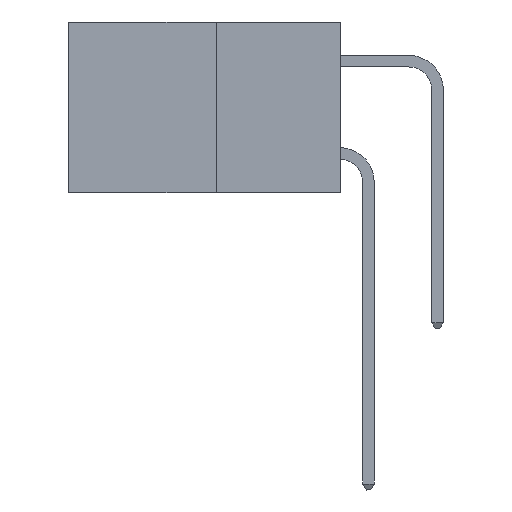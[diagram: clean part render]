
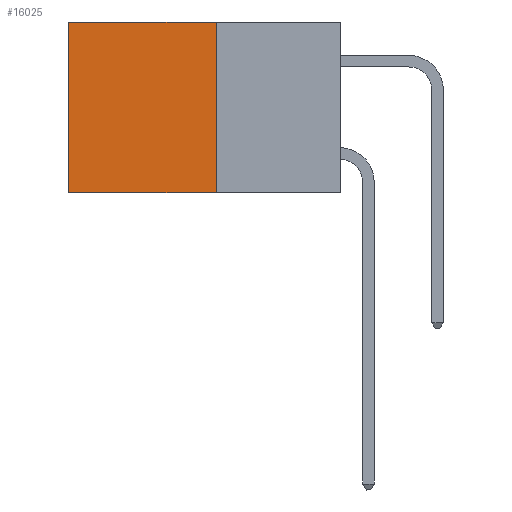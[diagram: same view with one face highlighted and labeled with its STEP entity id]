
A CAD part, left-side view. The second image highlights one B-rep face of the part: STEP entity #16025.
In plain terms, the highlighted planar face has unit normal (-1, 0, 0).
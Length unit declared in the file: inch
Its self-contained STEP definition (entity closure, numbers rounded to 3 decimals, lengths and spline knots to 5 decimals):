
#221 = EDGE_LOOP ( 'NONE', ( #6237, #7981, #3574, #17162 ) ) ;
#308 = CARTESIAN_POINT ( 'NONE',  ( 0.277, 0.59, -0.37 ) ) ;
#577 = EDGE_CURVE ( 'NONE', #3611, #1436, #14157, .T. ) ;
#1436 = VERTEX_POINT ( 'NONE', #17372 ) ;
#3574 = ORIENTED_EDGE ( 'NONE', *, *, #18549, .F. ) ;
#3611 = VERTEX_POINT ( 'NONE', #19410 ) ;
#4179 = DIRECTION ( 'NONE',  ( 0., 0., -1. ) ) ;
#4220 = DIRECTION ( 'NONE',  ( 1., 0., 0. ) ) ;
#4270 = PLANE ( 'NONE',  #16732 ) ;
#4299 = CARTESIAN_POINT ( 'NONE',  ( 0.277, 0.27, -0.37 ) ) ;
#4563 = EDGE_CURVE ( 'NONE', #4856, #1436, #8971, .T. ) ;
#4856 = VERTEX_POINT ( 'NONE', #14349 ) ;
#5514 = VECTOR ( 'NONE', #19115, 39.37008 ) ;
#5654 = VERTEX_POINT ( 'NONE', #15924 ) ;
#6237 = ORIENTED_EDGE ( 'NONE', *, *, #577, .T. ) ;
#6340 = FACE_OUTER_BOUND ( 'NONE', #221, .T. ) ;
#7776 = CARTESIAN_POINT ( 'NONE',  ( 0.277, 0.27, -0.37 ) ) ;
#7947 = CARTESIAN_POINT ( 'NONE',  ( 0.277, 0.27, -0.37 ) ) ;
#7981 = ORIENTED_EDGE ( 'NONE', *, *, #4563, .F. ) ;
#8590 = EDGE_CURVE ( 'NONE', #5654, #3611, #17774, .T. ) ;
#8971 = LINE ( 'NONE', #7776, #9439 ) ;
#8977 = DIRECTION ( 'NONE',  ( 0., 1., 0. ) ) ;
#9439 = VECTOR ( 'NONE', #16878, 39.37008 ) ;
#9458 = DIRECTION ( 'NONE',  ( 0., 0., -1. ) ) ;
#11848 = LINE ( 'NONE', #7947, #19123 ) ;
#13586 = VECTOR ( 'NONE', #8977, 39.37008 ) ;
#14157 = LINE ( 'NONE', #308, #5514 ) ;
#14349 = CARTESIAN_POINT ( 'NONE',  ( 0.277, 0.27, -0.37 ) ) ;
#15013 = CARTESIAN_POINT ( 'NONE',  ( 0.277, 0.27, 0. ) ) ;
#15924 = CARTESIAN_POINT ( 'NONE',  ( 0.277, 0.27, 0. ) ) ;
#16025 = ADVANCED_FACE ( 'NONE', ( #6340 ), #4270, .F. ) ;
#16732 = AXIS2_PLACEMENT_3D ( 'NONE', #4299, #4220, #4179 ) ;
#16878 = DIRECTION ( 'NONE',  ( 0., 1., 0. ) ) ;
#17162 = ORIENTED_EDGE ( 'NONE', *, *, #8590, .T. ) ;
#17372 = CARTESIAN_POINT ( 'NONE',  ( 0.277, 0.59, -0.37 ) ) ;
#17774 = LINE ( 'NONE', #15013, #13586 ) ;
#18549 = EDGE_CURVE ( 'NONE', #5654, #4856, #11848, .T. ) ;
#19115 = DIRECTION ( 'NONE',  ( 0., 0., -1. ) ) ;
#19123 = VECTOR ( 'NONE', #9458, 39.37008 ) ;
#19410 = CARTESIAN_POINT ( 'NONE',  ( 0.277, 0.59, 0. ) ) ;
